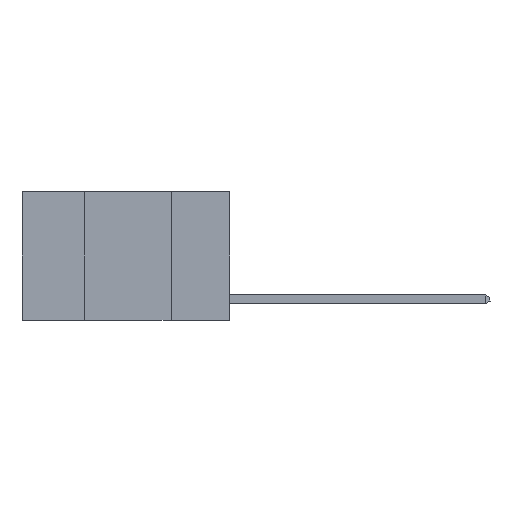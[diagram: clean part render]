
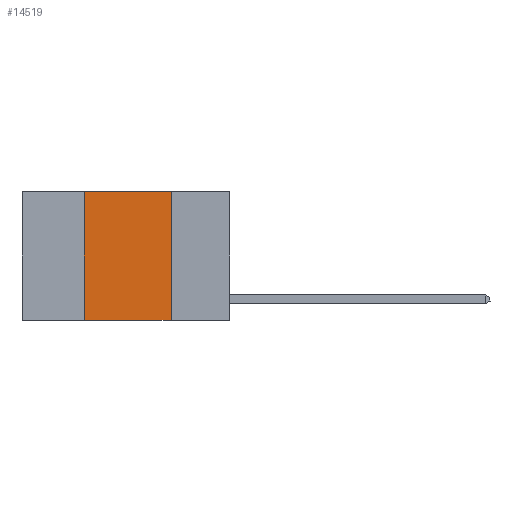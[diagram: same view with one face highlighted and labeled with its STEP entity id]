
A CAD part, left-side view. The second image highlights one B-rep face of the part: STEP entity #14519.
In plain terms, the highlighted planar face has unit normal (-1, 0, 0).
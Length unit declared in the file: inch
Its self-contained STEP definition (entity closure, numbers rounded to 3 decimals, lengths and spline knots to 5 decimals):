
#58 = CARTESIAN_POINT ( 'NONE',  ( 0., 0.17, 0. ) ) ;
#145 = EDGE_CURVE ( 'NONE', #9748, #11271, #6327, .T. ) ;
#175 = DIRECTION ( 'NONE',  ( 0., 0., 1. ) ) ;
#227 = CARTESIAN_POINT ( 'NONE',  ( 0., 0.17, -0.37 ) ) ;
#243 = VECTOR ( 'NONE', #15151, 39.37008 ) ;
#592 = EDGE_CURVE ( 'NONE', #11271, #16431, #17544, .T. ) ;
#1354 = ORIENTED_EDGE ( 'NONE', *, *, #145, .F. ) ;
#1896 = PLANE ( 'NONE',  #11467 ) ;
#3640 = VECTOR ( 'NONE', #6456, 39.37008 ) ;
#5929 = DIRECTION ( 'NONE',  ( 1., 0., 0. ) ) ;
#6327 = LINE ( 'NONE', #22489, #26126 ) ;
#6456 = DIRECTION ( 'NONE',  ( 0., 0., -1. ) ) ;
#8021 = DIRECTION ( 'NONE',  ( 0., 0., -1. ) ) ;
#9748 = VERTEX_POINT ( 'NONE', #21849 ) ;
#10338 = CARTESIAN_POINT ( 'NONE',  ( 0., 0.17, 0. ) ) ;
#11116 = LINE ( 'NONE', #16097, #25748 ) ;
#11271 = VERTEX_POINT ( 'NONE', #16200 ) ;
#11467 = AXIS2_PLACEMENT_3D ( 'NONE', #23963, #5929, #8021 ) ;
#13809 = VERTEX_POINT ( 'NONE', #227 ) ;
#14519 = ADVANCED_FACE ( 'NONE', ( #20291 ), #1896, .F. ) ;
#14786 = ORIENTED_EDGE ( 'NONE', *, *, #15223, .T. ) ;
#15151 = DIRECTION ( 'NONE',  ( 0., -1., 0. ) ) ;
#15223 = EDGE_CURVE ( 'NONE', #9748, #13809, #11116, .T. ) ;
#15643 = CARTESIAN_POINT ( 'NONE',  ( 0., 0.6, 0. ) ) ;
#16044 = EDGE_CURVE ( 'NONE', #16431, #13809, #17149, .T. ) ;
#16097 = CARTESIAN_POINT ( 'NONE',  ( 0., 0.6, -0.37 ) ) ;
#16200 = CARTESIAN_POINT ( 'NONE',  ( 0., 0.42, 0. ) ) ;
#16431 = VERTEX_POINT ( 'NONE', #58 ) ;
#17149 = LINE ( 'NONE', #10338, #3640 ) ;
#17544 = LINE ( 'NONE', #15643, #243 ) ;
#18295 = EDGE_LOOP ( 'NONE', ( #21118, #19493, #1354, #14786 ) ) ;
#19493 = ORIENTED_EDGE ( 'NONE', *, *, #592, .F. ) ;
#20291 = FACE_OUTER_BOUND ( 'NONE', #18295, .T. ) ;
#21118 = ORIENTED_EDGE ( 'NONE', *, *, #16044, .F. ) ;
#21849 = CARTESIAN_POINT ( 'NONE',  ( 0., 0.42, -0.37 ) ) ;
#22008 = DIRECTION ( 'NONE',  ( 0., -1., 0. ) ) ;
#22489 = CARTESIAN_POINT ( 'NONE',  ( 0., 0.42, 0. ) ) ;
#23963 = CARTESIAN_POINT ( 'NONE',  ( 0., 0.6, 0. ) ) ;
#25748 = VECTOR ( 'NONE', #22008, 39.37008 ) ;
#26126 = VECTOR ( 'NONE', #175, 39.37008 ) ;
